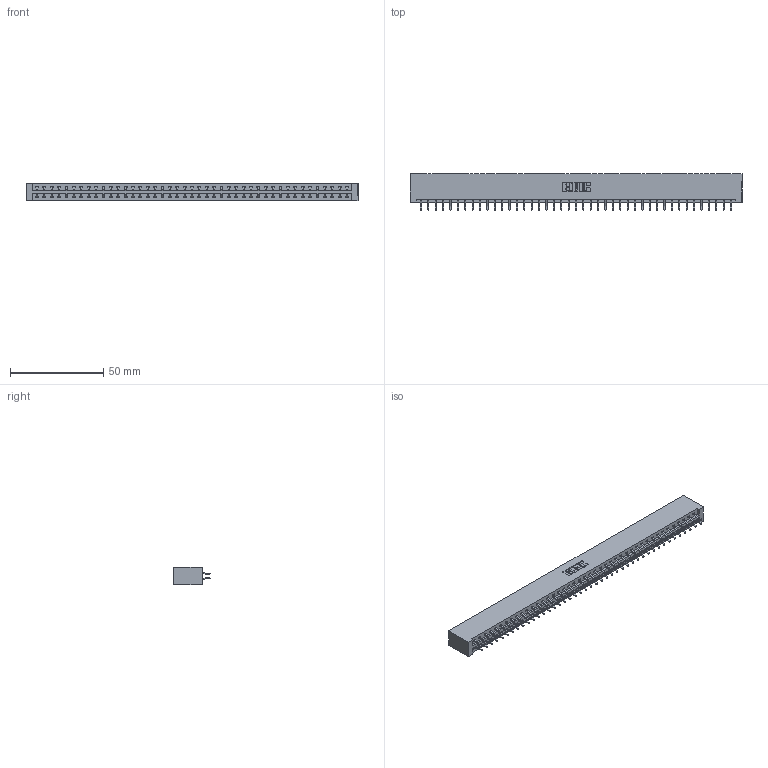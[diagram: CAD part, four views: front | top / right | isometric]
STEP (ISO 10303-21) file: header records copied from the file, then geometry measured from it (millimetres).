
FILE_DESCRIPTION (( 'STEP AP203' ), '1' );
FILE_NAME ('387-086-556-201.STEP', '2018-09-24T00:34:21', ( '' ), ( '' ), 'SwSTEP 2.0', 'SolidWorks 2016', '' );
FILE_SCHEMA (( 'CONFIG_CONTROL_DESIGN' ));
Length unit declared in the file: inch
Products named in the file (3): 387-086-556-201; 337 Part_No Mounting Lugs; 345-292-001_556 Tail
Assembly tree (87 placements, depth 2):
  387-086-556-201
    337 Part_No Mounting Lugs
    345-292-001_556 Tail  x86
Bounding box: 178.26 x 19.57 x 9.4 mm (x, y, z)
Volume: 19556.8 mm3; surface area: 22084.1 mm2
Topology: 87 solids, 87 shells, 5266 faces, 15681 edges, 10338 vertices
Faces by surface type: plane 3678, cylinder 1588
Entity records: 33153 total; most frequent: CARTESIAN_POINT 5598, ORIENTED_EDGE 5522, DIRECTION 4741, EDGE_CURVE 2761, VECTOR 2633, LINE 2633, VERTEX_POINT 1838, AXIS2_PLACEMENT_3D 1054
